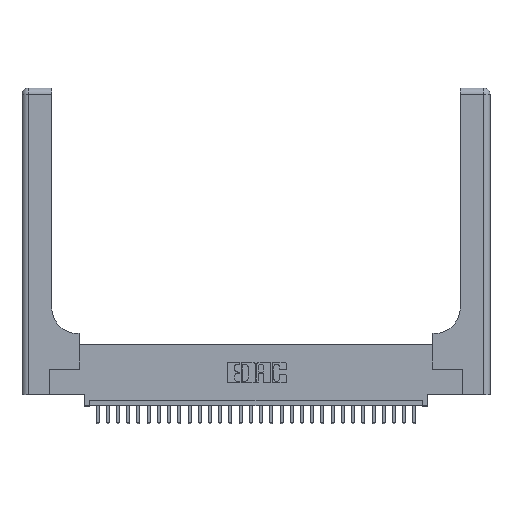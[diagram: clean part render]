
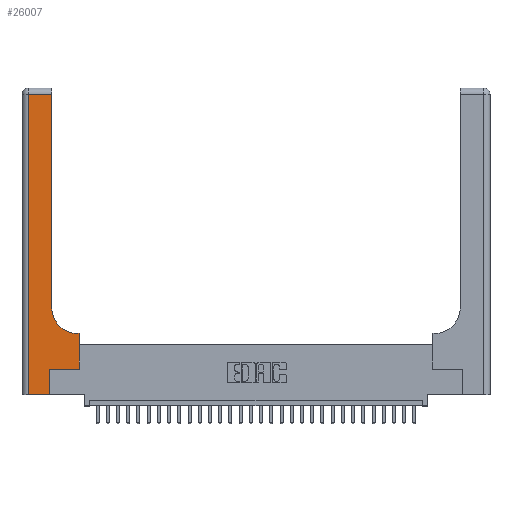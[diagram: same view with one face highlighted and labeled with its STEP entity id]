
A CAD part, top view. The second image highlights one B-rep face of the part: STEP entity #26007.
In plain terms, the highlighted planar face has unit normal (0, 0, 1).
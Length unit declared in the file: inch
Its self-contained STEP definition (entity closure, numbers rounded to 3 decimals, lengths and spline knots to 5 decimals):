
#55 = CARTESIAN_POINT ( 'NONE',  ( 0.5415, 0.85, 0.37 ) ) ;
#440 = ORIENTED_EDGE ( 'NONE', *, *, #11409, .T. ) ;
#450 = ORIENTED_EDGE ( 'NONE', *, *, #6964, .T. ) ;
#1455 = EDGE_CURVE ( 'NONE', #3077, #4376, #2784, .T. ) ;
#1614 = CARTESIAN_POINT ( 'NONE',  ( 0.5415, 0.6, 0.37 ) ) ;
#2229 = VECTOR ( 'NONE', #22487, 39.37008 ) ;
#2452 = DIRECTION ( 'NONE',  ( 1., 0., 0. ) ) ;
#2784 = LINE ( 'NONE', #26889, #27317 ) ;
#2931 = LINE ( 'NONE', #4805, #23370 ) ;
#3077 = VERTEX_POINT ( 'NONE', #21461 ) ;
#3166 = CARTESIAN_POINT ( 'NONE',  ( 0.5585, 0.25, 0.37 ) ) ;
#3789 = AXIS2_PLACEMENT_3D ( 'NONE', #7547, #21666, #24167 ) ;
#4019 = ORIENTED_EDGE ( 'NONE', *, *, #23603, .T. ) ;
#4086 = CARTESIAN_POINT ( 'NONE',  ( 0.06, 2.94, 0.37 ) ) ;
#4229 = ORIENTED_EDGE ( 'NONE', *, *, #12261, .T. ) ;
#4376 = VERTEX_POINT ( 'NONE', #1614 ) ;
#4805 = CARTESIAN_POINT ( 'NONE',  ( 0.269, 0.25, 0.37 ) ) ;
#4908 = CARTESIAN_POINT ( 'NONE',  ( 0.269, 0., 0.37 ) ) ;
#5042 = CARTESIAN_POINT ( 'NONE',  ( 0., 0., 0.37 ) ) ;
#5398 = EDGE_CURVE ( 'NONE', #10207, #3077, #15239, .T. ) ;
#5689 = DIRECTION ( 'NONE',  ( -1., 0., 0. ) ) ;
#6964 = EDGE_CURVE ( 'NONE', #25458, #10207, #2931, .T. ) ;
#7071 = CARTESIAN_POINT ( 'NONE',  ( 0.269, 0.25, 0.37 ) ) ;
#7547 = CARTESIAN_POINT ( 'NONE',  ( 0., 3., 0.37 ) ) ;
#7745 = PLANE ( 'NONE',  #3789 ) ;
#8123 = EDGE_CURVE ( 'NONE', #11543, #13312, #24404, .T. ) ;
#8234 = CARTESIAN_POINT ( 'NONE',  ( 0.5585, 0.25, 0.37 ) ) ;
#8682 = LINE ( 'NONE', #4908, #26916 ) ;
#8846 = CARTESIAN_POINT ( 'NONE',  ( 0.269, 0., 0.37 ) ) ;
#9625 = DIRECTION ( 'NONE',  ( 0., 0., -1. ) ) ;
#10207 = VERTEX_POINT ( 'NONE', #8234 ) ;
#11409 = EDGE_CURVE ( 'NONE', #15368, #11543, #12275, .T. ) ;
#11543 = VERTEX_POINT ( 'NONE', #4086 ) ;
#11962 = ORIENTED_EDGE ( 'NONE', *, *, #1455, .T. ) ;
#12216 = DIRECTION ( 'NONE',  ( 1., 0., 0. ) ) ;
#12261 = EDGE_CURVE ( 'NONE', #28859, #15368, #15137, .T. ) ;
#12275 = LINE ( 'NONE', #29847, #2229 ) ;
#13312 = VERTEX_POINT ( 'NONE', #30296 ) ;
#14172 = EDGE_CURVE ( 'NONE', #4376, #28859, #30809, .T. ) ;
#14616 = DIRECTION ( 'NONE',  ( 0., 1., 0. ) ) ;
#14893 = FACE_OUTER_BOUND ( 'NONE', #21186, .T. ) ;
#14994 = CARTESIAN_POINT ( 'NONE',  ( 0.2915, 0.85, 0.37 ) ) ;
#15137 = LINE ( 'NONE', #18632, #27060 ) ;
#15239 = LINE ( 'NONE', #3166, #26432 ) ;
#15368 = VERTEX_POINT ( 'NONE', #21344 ) ;
#16079 = ORIENTED_EDGE ( 'NONE', *, *, #5398, .T. ) ;
#16353 = DIRECTION ( 'NONE',  ( 0., 1., 0. ) ) ;
#16471 = DIRECTION ( 'NONE',  ( 0., -1., 0. ) ) ;
#16687 = CARTESIAN_POINT ( 'NONE',  ( 0.06, 3., 0.37 ) ) ;
#17701 = DIRECTION ( 'NONE',  ( 0., 1., 0. ) ) ;
#18632 = CARTESIAN_POINT ( 'NONE',  ( 0.2915, 3., 0.37 ) ) ;
#18928 = LINE ( 'NONE', #5042, #30166 ) ;
#19014 = VERTEX_POINT ( 'NONE', #8846 ) ;
#19541 = VECTOR ( 'NONE', #16471, 39.37008 ) ;
#21186 = EDGE_LOOP ( 'NONE', ( #4229, #440, #23499, #24250, #4019, #450, #16079, #11962, #29167 ) ) ;
#21344 = CARTESIAN_POINT ( 'NONE',  ( 0.2915, 2.94, 0.37 ) ) ;
#21461 = CARTESIAN_POINT ( 'NONE',  ( 0.5585, 0.6, 0.37 ) ) ;
#21666 = DIRECTION ( 'NONE',  ( 0., 0., -1. ) ) ;
#22487 = DIRECTION ( 'NONE',  ( -1., 0., 0. ) ) ;
#23370 = VECTOR ( 'NONE', #26100, 39.37008 ) ;
#23499 = ORIENTED_EDGE ( 'NONE', *, *, #8123, .T. ) ;
#23603 = EDGE_CURVE ( 'NONE', #19014, #25458, #8682, .T. ) ;
#24167 = DIRECTION ( 'NONE',  ( -1., 0., 0. ) ) ;
#24250 = ORIENTED_EDGE ( 'NONE', *, *, #26988, .T. ) ;
#24404 = LINE ( 'NONE', #16687, #19541 ) ;
#24488 = AXIS2_PLACEMENT_3D ( 'NONE', #55, #9625, #2452 ) ;
#25458 = VERTEX_POINT ( 'NONE', #7071 ) ;
#26007 = ADVANCED_FACE ( 'NONE', ( #14893 ), #7745, .F. ) ;
#26100 = DIRECTION ( 'NONE',  ( 1., 0., 0. ) ) ;
#26432 = VECTOR ( 'NONE', #14616, 39.37008 ) ;
#26889 = CARTESIAN_POINT ( 'NONE',  ( 0.2915, 0.6, 0.37 ) ) ;
#26916 = VECTOR ( 'NONE', #17701, 39.37008 ) ;
#26988 = EDGE_CURVE ( 'NONE', #13312, #19014, #18928, .T. ) ;
#27060 = VECTOR ( 'NONE', #16353, 39.37008 ) ;
#27317 = VECTOR ( 'NONE', #5689, 39.37008 ) ;
#28859 = VERTEX_POINT ( 'NONE', #14994 ) ;
#29167 = ORIENTED_EDGE ( 'NONE', *, *, #14172, .T. ) ;
#29847 = CARTESIAN_POINT ( 'NONE',  ( 0., 2.94, 0.37 ) ) ;
#30166 = VECTOR ( 'NONE', #12216, 39.37008 ) ;
#30296 = CARTESIAN_POINT ( 'NONE',  ( 0.06, 0., 0.37 ) ) ;
#30809 = CIRCLE ( 'NONE', #24488, 0.25 ) ;
